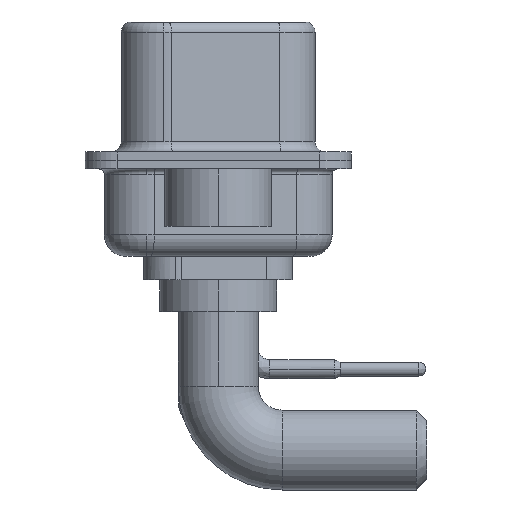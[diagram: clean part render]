
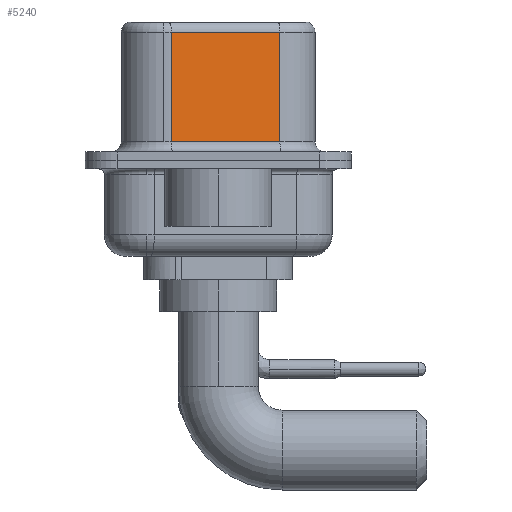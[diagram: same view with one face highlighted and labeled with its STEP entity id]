
A CAD part, left-side view. The second image highlights one B-rep face of the part: STEP entity #5240.
In plain terms, the highlighted planar face has unit normal (-0.985, -0.174, 0).
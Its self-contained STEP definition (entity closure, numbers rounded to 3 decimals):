
#799 = AXIS2_PLACEMENT_3D ( 'NONE', #24047, #20270, #6875 ) ;
#1053 = EDGE_LOOP ( 'NONE', ( #8734, #13113, #11490, #13468 ) ) ;
#1075 = CARTESIAN_POINT ( 'NONE',  ( 3.68, 2.203, 6.02 ) ) ;
#1100 = CARTESIAN_POINT ( 'NONE',  ( 4.58, -2.897, 0.9 ) ) ;
#1995 = EDGE_CURVE ( 'NONE', #5545, #17358, #13202, .T. ) ;
#3725 = EDGE_CURVE ( 'NONE', #17358, #5446, #15786, .T. ) ;
#4939 = DIRECTION ( 'NONE',  ( 0.174, -0.985, 0. ) ) ;
#5240 = ADVANCED_FACE ( 'NONE', ( #10877 ), #22276, .F. ) ;
#5446 = VERTEX_POINT ( 'NONE', #9385 ) ;
#5537 = VECTOR ( 'NONE', #18955, 1000. ) ;
#5545 = VERTEX_POINT ( 'NONE', #15764 ) ;
#6875 = DIRECTION ( 'NONE',  ( -0.174, 0.985, 0. ) ) ;
#6942 = CARTESIAN_POINT ( 'NONE',  ( 4.58, -2.897, 0.9 ) ) ;
#8692 = LINE ( 'NONE', #6942, #10575 ) ;
#8734 = ORIENTED_EDGE ( 'NONE', *, *, #20419, .F. ) ;
#9385 = CARTESIAN_POINT ( 'NONE',  ( 3.68, 2.203, 0.9 ) ) ;
#10575 = VECTOR ( 'NONE', #4939, 1000. ) ;
#10877 = FACE_OUTER_BOUND ( 'NONE', #1053, .T. ) ;
#11490 = ORIENTED_EDGE ( 'NONE', *, *, #3725, .T. ) ;
#12265 = DIRECTION ( 'NONE',  ( 0., 0., -1. ) ) ;
#13064 = LINE ( 'NONE', #19073, #18642 ) ;
#13113 = ORIENTED_EDGE ( 'NONE', *, *, #1995, .T. ) ;
#13202 = LINE ( 'NONE', #22465, #5537 ) ;
#13468 = ORIENTED_EDGE ( 'NONE', *, *, #19157, .T. ) ;
#14747 = VECTOR ( 'NONE', #12265, 1000. ) ;
#15542 = CARTESIAN_POINT ( 'NONE',  ( 3.68, 2.203, 6.52 ) ) ;
#15764 = CARTESIAN_POINT ( 'NONE',  ( 4.58, -2.897, 6.02 ) ) ;
#15786 = LINE ( 'NONE', #15542, #14747 ) ;
#17358 = VERTEX_POINT ( 'NONE', #1075 ) ;
#18642 = VECTOR ( 'NONE', #20959, 1000. ) ;
#18955 = DIRECTION ( 'NONE',  ( -0.174, 0.985, 0. ) ) ;
#19073 = CARTESIAN_POINT ( 'NONE',  ( 4.58, -2.897, 6.52 ) ) ;
#19157 = EDGE_CURVE ( 'NONE', #5446, #19876, #8692, .T. ) ;
#19876 = VERTEX_POINT ( 'NONE', #1100 ) ;
#20270 = DIRECTION ( 'NONE',  ( 0.985, 0.174, 0. ) ) ;
#20419 = EDGE_CURVE ( 'NONE', #5545, #19876, #13064, .T. ) ;
#20959 = DIRECTION ( 'NONE',  ( 0., 0., -1. ) ) ;
#22276 = PLANE ( 'NONE',  #799 ) ;
#22465 = CARTESIAN_POINT ( 'NONE',  ( 4.58, -2.897, 6.02 ) ) ;
#24047 = CARTESIAN_POINT ( 'NONE',  ( 4.58, -2.897, 6.52 ) ) ;
